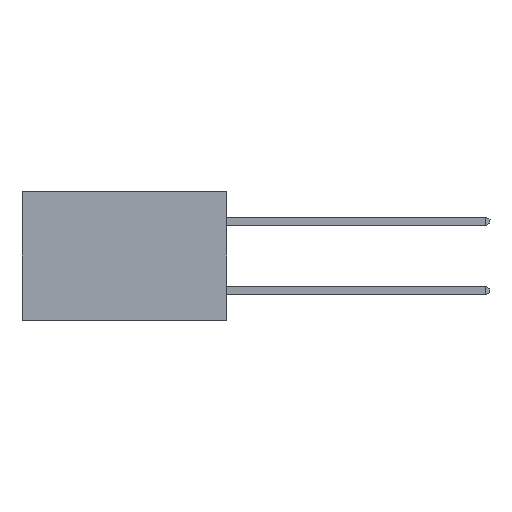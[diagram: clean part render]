
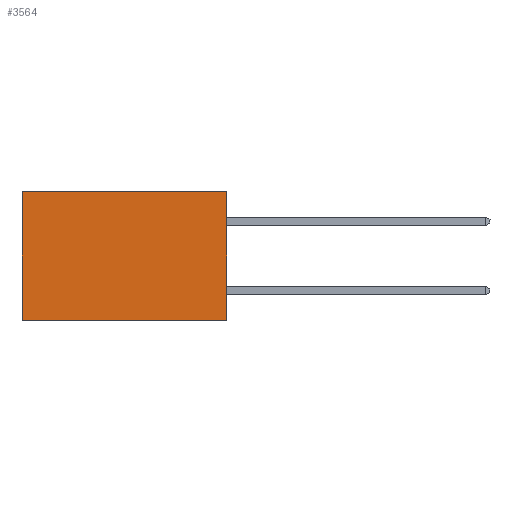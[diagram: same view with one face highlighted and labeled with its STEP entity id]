
A CAD part, left-side view. The second image highlights one B-rep face of the part: STEP entity #3564.
In plain terms, the highlighted planar face has unit normal (-1, 0, 0).
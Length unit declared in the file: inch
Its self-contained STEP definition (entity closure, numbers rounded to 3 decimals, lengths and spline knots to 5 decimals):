
#7 = DIRECTION ( 'NONE',  ( 0., 0., -1. ) ) ;
#30 = DIRECTION ( 'NONE',  ( 1., 0., 0. ) ) ;
#69 = PLANE ( 'NONE',  #4143 ) ;
#74 = CARTESIAN_POINT ( 'NONE',  ( 0.277, 0., -0.37 ) ) ;
#200 = DIRECTION ( 'NONE',  ( 0., 0., -1. ) ) ;
#236 = VERTEX_POINT ( 'NONE', #5083 ) ;
#432 = FACE_OUTER_BOUND ( 'NONE', #5594, .T. ) ;
#479 = EDGE_CURVE ( 'NONE', #2109, #1052, #3384, .T. ) ;
#512 = EDGE_CURVE ( 'NONE', #6851, #2109, #4454, .T. ) ;
#897 = DIRECTION ( 'NONE',  ( 0., 0., -1. ) ) ;
#1052 = VERTEX_POINT ( 'NONE', #6172 ) ;
#1127 = DIRECTION ( 'NONE',  ( 0., 1., 0. ) ) ;
#1193 = CARTESIAN_POINT ( 'NONE',  ( 0.277, 0., 0. ) ) ;
#1291 = EDGE_CURVE ( 'NONE', #236, #1052, #3527, .T. ) ;
#1412 = VECTOR ( 'NONE', #1512, 39.37008 ) ;
#1512 = DIRECTION ( 'NONE',  ( 0., 1., 0. ) ) ;
#1698 = CARTESIAN_POINT ( 'NONE',  ( 0.277, 0., 0. ) ) ;
#1915 = CARTESIAN_POINT ( 'NONE',  ( 0.277, 0., -0.37 ) ) ;
#2109 = VERTEX_POINT ( 'NONE', #6602 ) ;
#2731 = VECTOR ( 'NONE', #200, 39.37008 ) ;
#2788 = VECTOR ( 'NONE', #1127, 39.37008 ) ;
#3026 = CARTESIAN_POINT ( 'NONE',  ( 0.277, 0.59, -0.37 ) ) ;
#3289 = ORIENTED_EDGE ( 'NONE', *, *, #1291, .T. ) ;
#3353 = ORIENTED_EDGE ( 'NONE', *, *, #5042, .T. ) ;
#3384 = LINE ( 'NONE', #6057, #1412 ) ;
#3527 = LINE ( 'NONE', #3026, #6401 ) ;
#3564 = ADVANCED_FACE ( 'NONE', ( #432 ), #69, .F. ) ;
#4143 = AXIS2_PLACEMENT_3D ( 'NONE', #74, #30, #7 ) ;
#4454 = LINE ( 'NONE', #1915, #2731 ) ;
#4511 = ORIENTED_EDGE ( 'NONE', *, *, #512, .F. ) ;
#5042 = EDGE_CURVE ( 'NONE', #6851, #236, #7258, .T. ) ;
#5083 = CARTESIAN_POINT ( 'NONE',  ( 0.277, 0.59, 0. ) ) ;
#5594 = EDGE_LOOP ( 'NONE', ( #3289, #5795, #4511, #3353 ) ) ;
#5795 = ORIENTED_EDGE ( 'NONE', *, *, #479, .F. ) ;
#6057 = CARTESIAN_POINT ( 'NONE',  ( 0.277, 0., -0.37 ) ) ;
#6172 = CARTESIAN_POINT ( 'NONE',  ( 0.277, 0.59, -0.37 ) ) ;
#6401 = VECTOR ( 'NONE', #897, 39.37008 ) ;
#6602 = CARTESIAN_POINT ( 'NONE',  ( 0.277, 0., -0.37 ) ) ;
#6851 = VERTEX_POINT ( 'NONE', #1698 ) ;
#7258 = LINE ( 'NONE', #1193, #2788 ) ;
